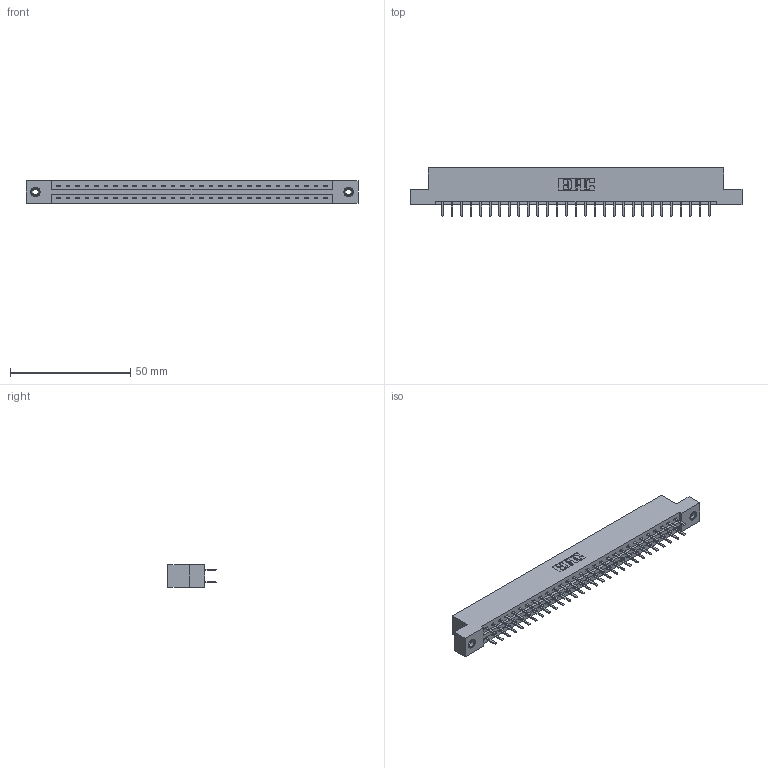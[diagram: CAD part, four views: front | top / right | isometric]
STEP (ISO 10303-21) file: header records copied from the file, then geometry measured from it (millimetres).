
FILE_DESCRIPTION (( 'STEP AP203' ), '1' );
FILE_NAME ('387-058-520-208.STEP', '2019-10-19T08:18:49', ( '' ), ( '' ), 'SwSTEP 2.0', 'SolidWorks 2016', '' );
FILE_SCHEMA (( 'CONFIG_CONTROL_DESIGN' ));
Length unit declared in the file: inch
Products named in the file (4): 387-058-520-208; 337 Part_Flush Mounting Lugs - 0.156 Dia-TI; 345-250-001_345-250-003-102; 345-292-001_345-293-120
Assembly tree (61 placements, depth 2):
  387-058-520-208
    337 Part_Flush Mounting Lugs - 0.156 Dia-TI
    345-292-001_345-293-120  x58
    345-250-001_345-250-003-102  x2
Bounding box: 137.92 x 20.02 x 9.4 mm (x, y, z)
Volume: 14330.3 mm3; surface area: 16025.3 mm2
Topology: 61 solids, 61 shells, 3538 faces, 10249 edges, 6670 vertices
Faces by surface type: plane 2422, cylinder 1100, cone 12, torus 4
Entity records: 25466 total; most frequent: CARTESIAN_POINT 4293, ORIENTED_EDGE 4210, DIRECTION 3695, EDGE_CURVE 2105, LINE 1953, VECTOR 1953, VERTEX_POINT 1396, AXIS2_PLACEMENT_3D 871
